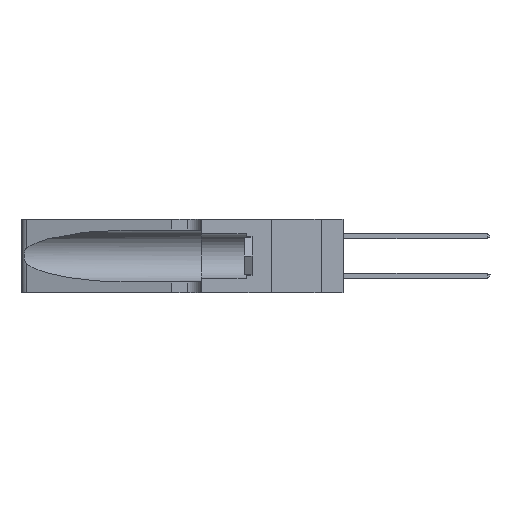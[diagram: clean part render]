
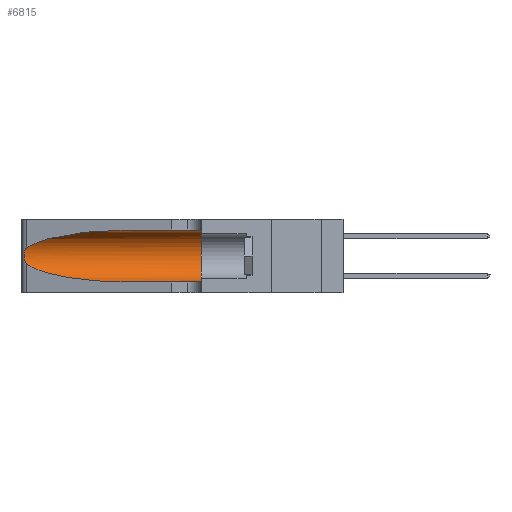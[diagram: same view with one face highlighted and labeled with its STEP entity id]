
A CAD part, left-side view. The second image highlights one B-rep face of the part: STEP entity #6815.
In plain terms, the highlighted cylindrical face has radius 3.308 mm (diameter 6.617 mm), a partial arc.
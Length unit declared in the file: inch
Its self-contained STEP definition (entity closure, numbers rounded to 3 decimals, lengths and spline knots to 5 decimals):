
#143 = CARTESIAN_POINT ( 'NONE',  ( 0.25856, 1.23593, 0.16098 ) ) ;
#393 = CARTESIAN_POINT ( 'NONE',  ( 0.25487, 1.22718, 0.22369 ) ) ;
#2536 = CARTESIAN_POINT ( 'NONE',  ( 0.25487, 1.22718, 0.22369 ) ) ;
#2860 = EDGE_CURVE ( 'NONE', #7497, #12013, #15587, .T. ) ;
#3606 = LINE ( 'NONE', #17312, #29120 ) ;
#4620 = EDGE_CURVE ( 'NONE', #12013, #15659, #3606, .T. ) ;
#4799 = EDGE_CURVE ( 'NONE', #16639, #15460, #9750, .T. ) ;
#5693 = CARTESIAN_POINT ( 'NONE',  ( 0.25639, 1.23184, 0.21858 ) ) ;
#5815 = CARTESIAN_POINT ( 'NONE',  ( 0.26075, 1.23896, 0.178 ) ) ;
#6407 = EDGE_CURVE ( 'NONE', #31768, #15659, #24988, .T. ) ;
#6708 = DIRECTION ( 'NONE',  ( 0., 0., 1. ) ) ;
#6728 = EDGE_CURVE ( 'NONE', #16639, #31768, #22763, .T. ) ;
#6815 = ADVANCED_FACE ( 'NONE', ( #34621 ), #30244, .F. ) ;
#7418 = DIRECTION ( 'NONE',  ( 0., -1., 0. ) ) ;
#7497 = VERTEX_POINT ( 'NONE', #8847 ) ;
#7829 = VECTOR ( 'NONE', #33822, 39.37008 ) ;
#8211 = CARTESIAN_POINT ( 'NONE',  ( 0.25487, 1.22718, 0.22369 ) ) ;
#8847 = CARTESIAN_POINT ( 'NONE',  ( 0.25487, 1.22718, 0.14631 ) ) ;
#9319 = ORIENTED_EDGE ( 'NONE', *, *, #6728, .F. ) ;
#9750 =( BOUNDED_CURVE ( )  B_SPLINE_CURVE ( 3, ( #25376, #19217, #16490, #2536 ),
 .UNSPECIFIED., .F., .F. ) 
 B_SPLINE_CURVE_WITH_KNOTS ( ( 4, 4 ),
 ( 1.5708, 2.84003 ),
 .UNSPECIFIED. ) 
 CURVE ( )  GEOMETRIC_REPRESENTATION_ITEM ( )  RATIONAL_B_SPLINE_CURVE ( ( 1., 0.87, 0.87, 1. ) ) 
 REPRESENTATION_ITEM ( '' )  );
#11565 = CARTESIAN_POINT ( 'NONE',  ( 0.25789, 1.23486, 0.15765 ) ) ;
#12013 = VERTEX_POINT ( 'NONE', #26818 ) ;
#14288 = CARTESIAN_POINT ( 'NONE',  ( 0.2373, 1.15595, 0.08982 ) ) ;
#15044 = CARTESIAN_POINT ( 'NONE',  ( 0.1305, 0.35, 0.31525 ) ) ;
#15460 = VERTEX_POINT ( 'NONE', #8211 ) ;
#15587 =( BOUNDED_CURVE ( )  B_SPLINE_CURVE ( 3, ( #30683, #14288, #33871, #24172 ),
 .UNSPECIFIED., .F., .T. ) 
 B_SPLINE_CURVE_WITH_KNOTS ( ( 4, 4 ),
 ( 3.44316, 4.71239 ),
 .UNSPECIFIED. ) 
 CURVE ( )  GEOMETRIC_REPRESENTATION_ITEM ( )  RATIONAL_B_SPLINE_CURVE ( ( 1., 0.87, 0.87, 1. ) ) 
 REPRESENTATION_ITEM ( '' )  );
#15659 = VERTEX_POINT ( 'NONE', #29312 ) ;
#16490 = CARTESIAN_POINT ( 'NONE',  ( 0.2373, 1.15595, 0.28018 ) ) ;
#16639 = VERTEX_POINT ( 'NONE', #23034 ) ;
#16934 = DIRECTION ( 'NONE',  ( 0., 0., -1. ) ) ;
#17186 = CARTESIAN_POINT ( 'NONE',  ( 0.25487, 1.22718, 0.14631 ) ) ;
#17215 = AXIS2_PLACEMENT_3D ( 'NONE', #29323, #21047, #6708 ) ;
#17308 = CARTESIAN_POINT ( 'NONE',  ( 0.25787, 1.23484, 0.2124 ) ) ;
#17312 = CARTESIAN_POINT ( 'NONE',  ( 0.1305, 1.61858, 0.05475 ) ) ;
#18551 = ORIENTED_EDGE ( 'NONE', *, *, #2860, .T. ) ;
#19217 = CARTESIAN_POINT ( 'NONE',  ( 0.18966, 0.96281, 0.31525 ) ) ;
#19672 = CARTESIAN_POINT ( 'NONE',  ( 0.25555, 1.22994, 0.2215 ) ) ;
#19783 = CARTESIAN_POINT ( 'NONE',  ( 0.25854, 1.2359, 0.20912 ) ) ;
#20146 = CARTESIAN_POINT ( 'NONE',  ( 0.1305, 1.61858, 0.31525 ) ) ;
#20654 = ORIENTED_EDGE ( 'NONE', *, *, #6407, .F. ) ;
#21047 = DIRECTION ( 'NONE',  ( 0., 1., 0. ) ) ;
#21579 = ORIENTED_EDGE ( 'NONE', *, *, #4620, .T. ) ;
#22763 = LINE ( 'NONE', #20146, #7829 ) ;
#22988 = CARTESIAN_POINT ( 'NONE',  ( 0.1305, 1.61858, 0.185 ) ) ;
#23034 = CARTESIAN_POINT ( 'NONE',  ( 0.1305, 0.72297, 0.31525 ) ) ;
#23387 = EDGE_CURVE ( 'NONE', #15460, #7497, #24395, .T. ) ;
#24172 = CARTESIAN_POINT ( 'NONE',  ( 0.1305, 0.72297, 0.05475 ) ) ;
#24395 = B_SPLINE_CURVE_WITH_KNOTS ( 'NONE', 3,
 ( #393, #19672, #5693, #17308, #19783, #28329, #31361, #5815, #28571, #143, #11565, #25699, #34059, #17186 ),
 .UNSPECIFIED., .F., .F.,
 ( 4, 2, 2, 2, 2, 2, 4 ),
 ( 0., 0.00027, 0.00053, 0.00107, 0.0016, 0.00187, 0.00214 ),
 .UNSPECIFIED. ) ;
#24988 = CIRCLE ( 'NONE', #17215, 0.13025 ) ;
#25376 = CARTESIAN_POINT ( 'NONE',  ( 0.1305, 0.72297, 0.31525 ) ) ;
#25699 = CARTESIAN_POINT ( 'NONE',  ( 0.25639, 1.23186, 0.15144 ) ) ;
#25716 = EDGE_LOOP ( 'NONE', ( #35186, #35573, #18551, #21579, #20654, #9319 ) ) ;
#26818 = CARTESIAN_POINT ( 'NONE',  ( 0.1305, 0.72297, 0.05475 ) ) ;
#28205 = DIRECTION ( 'NONE',  ( 0., -1., 0. ) ) ;
#28329 = CARTESIAN_POINT ( 'NONE',  ( 0.26018, 1.23835, 0.19895 ) ) ;
#28571 = CARTESIAN_POINT ( 'NONE',  ( 0.26017, 1.23833, 0.17102 ) ) ;
#29120 = VECTOR ( 'NONE', #7418, 39.37008 ) ;
#29312 = CARTESIAN_POINT ( 'NONE',  ( 0.1305, 0.35, 0.05475 ) ) ;
#29323 = CARTESIAN_POINT ( 'NONE',  ( 0.1305, 0.35, 0.185 ) ) ;
#30244 = CYLINDRICAL_SURFACE ( 'NONE', #36277, 0.13025 ) ;
#30683 = CARTESIAN_POINT ( 'NONE',  ( 0.25487, 1.22718, 0.14631 ) ) ;
#31361 = CARTESIAN_POINT ( 'NONE',  ( 0.26075, 1.23896, 0.19203 ) ) ;
#31768 = VERTEX_POINT ( 'NONE', #15044 ) ;
#33822 = DIRECTION ( 'NONE',  ( 0., -1., 0. ) ) ;
#33871 = CARTESIAN_POINT ( 'NONE',  ( 0.18966, 0.96281, 0.05475 ) ) ;
#34059 = CARTESIAN_POINT ( 'NONE',  ( 0.25555, 1.22993, 0.14849 ) ) ;
#34621 = FACE_OUTER_BOUND ( 'NONE', #25716, .T. ) ;
#35186 = ORIENTED_EDGE ( 'NONE', *, *, #4799, .T. ) ;
#35573 = ORIENTED_EDGE ( 'NONE', *, *, #23387, .T. ) ;
#36277 = AXIS2_PLACEMENT_3D ( 'NONE', #22988, #28205, #16934 ) ;
